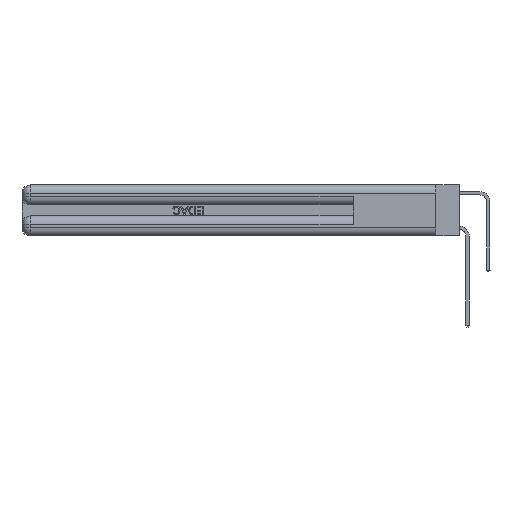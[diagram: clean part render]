
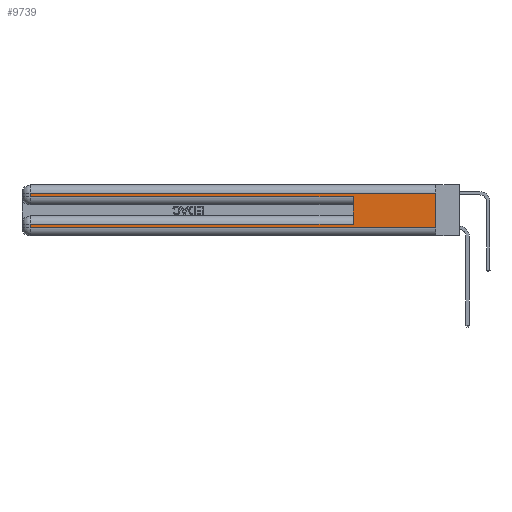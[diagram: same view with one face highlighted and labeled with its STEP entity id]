
A CAD part, left-side view. The second image highlights one B-rep face of the part: STEP entity #9739.
In plain terms, the highlighted planar face has unit normal (-1, 0, 0).
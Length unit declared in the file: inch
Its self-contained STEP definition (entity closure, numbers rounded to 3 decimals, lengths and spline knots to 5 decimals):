
#362 = EDGE_CURVE ( 'NONE', #19483, #19356, #9681, .T. ) ;
#1203 = CARTESIAN_POINT ( 'NONE',  ( 0., 0., 0.37 ) ) ;
#1307 = CARTESIAN_POINT ( 'NONE',  ( 0., 0.6, 0.285 ) ) ;
#1534 = VECTOR ( 'NONE', #3868, 39.37008 ) ;
#2008 = EDGE_CURVE ( 'NONE', #9260, #14828, #7917, .T. ) ;
#3783 = CARTESIAN_POINT ( 'NONE',  ( 0., 0., 0.06 ) ) ;
#3810 = ORIENTED_EDGE ( 'NONE', *, *, #15873, .T. ) ;
#3868 = DIRECTION ( 'NONE',  ( 0., 0., 1. ) ) ;
#3887 = FACE_OUTER_BOUND ( 'NONE', #26585, .T. ) ;
#3941 = VECTOR ( 'NONE', #9147, 39.37008 ) ;
#4415 = ORIENTED_EDGE ( 'NONE', *, *, #4898, .T. ) ;
#4787 = ORIENTED_EDGE ( 'NONE', *, *, #2008, .T. ) ;
#4898 = EDGE_CURVE ( 'NONE', #19314, #19356, #22282, .T. ) ;
#6240 = CARTESIAN_POINT ( 'NONE',  ( 0., 2.94, 0.06 ) ) ;
#6623 = EDGE_CURVE ( 'NONE', #19483, #19971, #31142, .T. ) ;
#7509 = CARTESIAN_POINT ( 'NONE',  ( 0., 2.94, 0.285 ) ) ;
#7917 = LINE ( 'NONE', #10749, #33448 ) ;
#8251 = DIRECTION ( 'NONE',  ( 0., -1., 0. ) ) ;
#8330 = VECTOR ( 'NONE', #30774, 39.37008 ) ;
#9040 = CARTESIAN_POINT ( 'NONE',  ( 0., 0., 0.285 ) ) ;
#9147 = DIRECTION ( 'NONE',  ( 0., 1., 0. ) ) ;
#9260 = VERTEX_POINT ( 'NONE', #6240 ) ;
#9681 = LINE ( 'NONE', #31118, #1534 ) ;
#9739 = ADVANCED_FACE ( 'NONE', ( #3887 ), #22597, .F. ) ;
#10617 = VECTOR ( 'NONE', #24285, 39.37008 ) ;
#10749 = CARTESIAN_POINT ( 'NONE',  ( 0., 0., 0.06 ) ) ;
#11164 = CARTESIAN_POINT ( 'NONE',  ( 0., 0., 0.31 ) ) ;
#11585 = DIRECTION ( 'NONE',  ( 0., 0., -1. ) ) ;
#13644 = AXIS2_PLACEMENT_3D ( 'NONE', #1203, #30239, #17122 ) ;
#14019 = VECTOR ( 'NONE', #11585, 39.37008 ) ;
#14301 = CARTESIAN_POINT ( 'NONE',  ( 0., 0., 0.085 ) ) ;
#14750 = LINE ( 'NONE', #30352, #14019 ) ;
#14828 = VERTEX_POINT ( 'NONE', #3783 ) ;
#15873 = EDGE_CURVE ( 'NONE', #19971, #9260, #23595, .T. ) ;
#16666 = ORIENTED_EDGE ( 'NONE', *, *, #362, .F. ) ;
#17101 = LINE ( 'NONE', #33411, #3941 ) ;
#17122 = DIRECTION ( 'NONE',  ( 0., 0., -1. ) ) ;
#18531 = ORIENTED_EDGE ( 'NONE', *, *, #23203, .F. ) ;
#18997 = VECTOR ( 'NONE', #19977, 39.37008 ) ;
#19305 = VECTOR ( 'NONE', #28560, 39.37008 ) ;
#19314 = VERTEX_POINT ( 'NONE', #7509 ) ;
#19345 = ORIENTED_EDGE ( 'NONE', *, *, #22799, .T. ) ;
#19356 = VERTEX_POINT ( 'NONE', #1307 ) ;
#19429 = VERTEX_POINT ( 'NONE', #28724 ) ;
#19483 = VERTEX_POINT ( 'NONE', #21080 ) ;
#19971 = VERTEX_POINT ( 'NONE', #32049 ) ;
#19977 = DIRECTION ( 'NONE',  ( 0., -1., 0. ) ) ;
#21080 = CARTESIAN_POINT ( 'NONE',  ( 0., 0.6, 0.085 ) ) ;
#22282 = LINE ( 'NONE', #9040, #18997 ) ;
#22597 = PLANE ( 'NONE',  #13644 ) ;
#22799 = EDGE_CURVE ( 'NONE', #32780, #19429, #17101, .T. ) ;
#23203 = EDGE_CURVE ( 'NONE', #32780, #14828, #14750, .T. ) ;
#23595 = LINE ( 'NONE', #26423, #10617 ) ;
#24285 = DIRECTION ( 'NONE',  ( 0., 0., -1. ) ) ;
#25887 = LINE ( 'NONE', #31767, #19305 ) ;
#26423 = CARTESIAN_POINT ( 'NONE',  ( 0., 2.94, 0.37 ) ) ;
#26585 = EDGE_LOOP ( 'NONE', ( #18531, #19345, #30323, #4415, #16666, #29729, #3810, #4787 ) ) ;
#28560 = DIRECTION ( 'NONE',  ( 0., 0., -1. ) ) ;
#28724 = CARTESIAN_POINT ( 'NONE',  ( 0., 2.94, 0.31 ) ) ;
#29729 = ORIENTED_EDGE ( 'NONE', *, *, #6623, .T. ) ;
#30239 = DIRECTION ( 'NONE',  ( 1., 0., 0. ) ) ;
#30323 = ORIENTED_EDGE ( 'NONE', *, *, #33919, .T. ) ;
#30352 = CARTESIAN_POINT ( 'NONE',  ( 0., 0., 0.37 ) ) ;
#30774 = DIRECTION ( 'NONE',  ( 0., 1., 0. ) ) ;
#31118 = CARTESIAN_POINT ( 'NONE',  ( 0., 0.6, 0.145 ) ) ;
#31142 = LINE ( 'NONE', #14301, #8330 ) ;
#31767 = CARTESIAN_POINT ( 'NONE',  ( 0., 2.94, 0.37 ) ) ;
#32049 = CARTESIAN_POINT ( 'NONE',  ( 0., 2.94, 0.085 ) ) ;
#32780 = VERTEX_POINT ( 'NONE', #11164 ) ;
#33411 = CARTESIAN_POINT ( 'NONE',  ( 0., 0., 0.31 ) ) ;
#33448 = VECTOR ( 'NONE', #8251, 39.37008 ) ;
#33919 = EDGE_CURVE ( 'NONE', #19429, #19314, #25887, .T. ) ;
